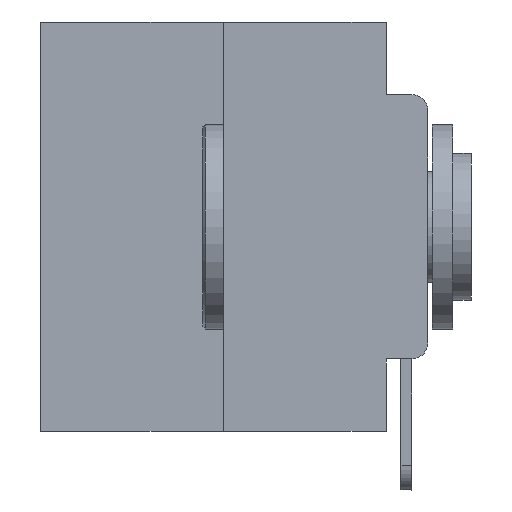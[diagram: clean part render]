
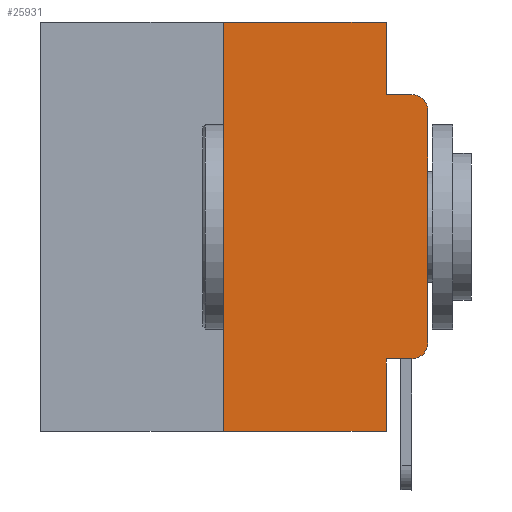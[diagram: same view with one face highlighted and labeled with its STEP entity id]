
A CAD part, left-side view. The second image highlights one B-rep face of the part: STEP entity #25931.
In plain terms, the highlighted planar face has unit normal (-1, 0, 0).
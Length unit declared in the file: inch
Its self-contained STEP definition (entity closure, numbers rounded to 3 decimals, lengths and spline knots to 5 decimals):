
#199 = ORIENTED_EDGE ( 'NONE', *, *, #8933, .F. ) ;
#407 = CARTESIAN_POINT ( 'NONE',  ( 0., 0.051, -0.5 ) ) ;
#454 = CARTESIAN_POINT ( 'NONE',  ( 0., 0.051, 0. ) ) ;
#742 = CARTESIAN_POINT ( 'NONE',  ( 0., 0.051, -0.4115 ) ) ;
#1163 = ORIENTED_EDGE ( 'NONE', *, *, #13655, .T. ) ;
#1267 = DIRECTION ( 'NONE',  ( -1., 0., 0. ) ) ;
#1526 = ORIENTED_EDGE ( 'NONE', *, *, #23392, .T. ) ;
#1685 = VECTOR ( 'NONE', #5749, 39.37008 ) ;
#1769 = DIRECTION ( 'NONE',  ( 0., -1., 0. ) ) ;
#1817 = DIRECTION ( 'NONE',  ( -1., 0., 0. ) ) ;
#2020 = VECTOR ( 'NONE', #12813, 39.37008 ) ;
#2674 = CARTESIAN_POINT ( 'NONE',  ( 0., 0., -0.3915 ) ) ;
#2781 = VERTEX_POINT ( 'NONE', #25508 ) ;
#3095 = EDGE_LOOP ( 'NONE', ( #1526, #18549, #21742, #27456, #24276, #199, #17093, #4495, #1163, #11969 ) ) ;
#3250 = DIRECTION ( 'NONE',  ( 0., 0., -1. ) ) ;
#3511 = CARTESIAN_POINT ( 'NONE',  ( 0., 0., -0.1085 ) ) ;
#3721 = DIRECTION ( 'NONE',  ( 1., 0., 0. ) ) ;
#3898 = VERTEX_POINT ( 'NONE', #15413 ) ;
#4325 = CARTESIAN_POINT ( 'NONE',  ( 0., 0.02, -0.4115 ) ) ;
#4481 = EDGE_CURVE ( 'NONE', #4596, #24447, #20565, .T. ) ;
#4495 = ORIENTED_EDGE ( 'NONE', *, *, #12337, .F. ) ;
#4596 = VERTEX_POINT ( 'NONE', #4325 ) ;
#5749 = DIRECTION ( 'NONE',  ( 0., -1., 0. ) ) ;
#5835 = DIRECTION ( 'NONE',  ( 0., 0., -1. ) ) ;
#5890 = CARTESIAN_POINT ( 'NONE',  ( 0., 0.02, -0.3915 ) ) ;
#6168 = CARTESIAN_POINT ( 'NONE',  ( 0., 0.02, -0.1085 ) ) ;
#6625 = DIRECTION ( 'NONE',  ( 0., 0., 1. ) ) ;
#7272 = VECTOR ( 'NONE', #23406, 39.37008 ) ;
#7619 = CIRCLE ( 'NONE', #13939, 0.02 ) ;
#8236 = LINE ( 'NONE', #26547, #24006 ) ;
#8284 = DIRECTION ( 'NONE',  ( 0., 0., -1. ) ) ;
#8599 = LINE ( 'NONE', #10998, #22497 ) ;
#8933 = EDGE_CURVE ( 'NONE', #17417, #26245, #14877, .T. ) ;
#9037 = LINE ( 'NONE', #454, #23569 ) ;
#9914 = FACE_OUTER_BOUND ( 'NONE', #3095, .T. ) ;
#10382 = DIRECTION ( 'NONE',  ( 0., 0., -1. ) ) ;
#10402 = CARTESIAN_POINT ( 'NONE',  ( 0., 0.051, 0. ) ) ;
#10444 = DIRECTION ( 'NONE',  ( 0., -1., 0. ) ) ;
#10998 = CARTESIAN_POINT ( 'NONE',  ( 0., 0., 0. ) ) ;
#11969 = ORIENTED_EDGE ( 'NONE', *, *, #4481, .T. ) ;
#12337 = EDGE_CURVE ( 'NONE', #20763, #17172, #9037, .T. ) ;
#12813 = DIRECTION ( 'NONE',  ( 0., 0., -1. ) ) ;
#13123 = CARTESIAN_POINT ( 'NONE',  ( 0., 0.473, -0.5 ) ) ;
#13205 = AXIS2_PLACEMENT_3D ( 'NONE', #14280, #3721, #5835 ) ;
#13655 = EDGE_CURVE ( 'NONE', #20763, #4596, #15368, .T. ) ;
#13803 = LINE ( 'NONE', #22341, #1685 ) ;
#13939 = AXIS2_PLACEMENT_3D ( 'NONE', #6168, #1817, #10382 ) ;
#14275 = CARTESIAN_POINT ( 'NONE',  ( 0., 0.051, 0. ) ) ;
#14280 = CARTESIAN_POINT ( 'NONE',  ( 0., 0.473, 0. ) ) ;
#14877 = LINE ( 'NONE', #23133, #7272 ) ;
#15304 = CARTESIAN_POINT ( 'NONE',  ( 0., 0.051, -0.4115 ) ) ;
#15368 = LINE ( 'NONE', #742, #25357 ) ;
#15406 = EDGE_CURVE ( 'NONE', #3898, #2781, #13803, .T. ) ;
#15413 = CARTESIAN_POINT ( 'NONE',  ( 0., 0.051, -0.0885 ) ) ;
#16130 = AXIS2_PLACEMENT_3D ( 'NONE', #5890, #1267, #8284 ) ;
#16665 = PLANE ( 'NONE',  #13205 ) ;
#17017 = LINE ( 'NONE', #10402, #2020 ) ;
#17093 = ORIENTED_EDGE ( 'NONE', *, *, #27704, .T. ) ;
#17172 = VERTEX_POINT ( 'NONE', #407 ) ;
#17417 = VERTEX_POINT ( 'NONE', #22321 ) ;
#17690 = VECTOR ( 'NONE', #10444, 39.37008 ) ;
#17782 = CARTESIAN_POINT ( 'NONE',  ( 0., 0.25, 0. ) ) ;
#18549 = ORIENTED_EDGE ( 'NONE', *, *, #20640, .T. ) ;
#19708 = DIRECTION ( 'NONE',  ( 0., -1., 0. ) ) ;
#20565 = CIRCLE ( 'NONE', #16130, 0.02 ) ;
#20640 = EDGE_CURVE ( 'NONE', #26744, #2781, #7619, .T. ) ;
#20763 = VERTEX_POINT ( 'NONE', #15304 ) ;
#21742 = ORIENTED_EDGE ( 'NONE', *, *, #15406, .F. ) ;
#22321 = CARTESIAN_POINT ( 'NONE',  ( 0., 0.25, -0.5 ) ) ;
#22341 = CARTESIAN_POINT ( 'NONE',  ( 0., 0.051, -0.0885 ) ) ;
#22497 = VECTOR ( 'NONE', #6625, 39.37008 ) ;
#23133 = CARTESIAN_POINT ( 'NONE',  ( 0., 0.25, 0. ) ) ;
#23211 = LINE ( 'NONE', #13123, #17690 ) ;
#23392 = EDGE_CURVE ( 'NONE', #24447, #26744, #8599, .T. ) ;
#23406 = DIRECTION ( 'NONE',  ( 0., 0., 1. ) ) ;
#23569 = VECTOR ( 'NONE', #3250, 39.37008 ) ;
#23985 = VERTEX_POINT ( 'NONE', #14275 ) ;
#24006 = VECTOR ( 'NONE', #1769, 39.37008 ) ;
#24276 = ORIENTED_EDGE ( 'NONE', *, *, #27109, .F. ) ;
#24447 = VERTEX_POINT ( 'NONE', #2674 ) ;
#25357 = VECTOR ( 'NONE', #19708, 39.37008 ) ;
#25508 = CARTESIAN_POINT ( 'NONE',  ( 0., 0.02, -0.0885 ) ) ;
#25931 = ADVANCED_FACE ( 'NONE', ( #9914 ), #16665, .F. ) ;
#26245 = VERTEX_POINT ( 'NONE', #17782 ) ;
#26547 = CARTESIAN_POINT ( 'NONE',  ( 0., 0.473, 0. ) ) ;
#26744 = VERTEX_POINT ( 'NONE', #3511 ) ;
#26955 = EDGE_CURVE ( 'NONE', #23985, #3898, #17017, .T. ) ;
#27109 = EDGE_CURVE ( 'NONE', #26245, #23985, #8236, .T. ) ;
#27456 = ORIENTED_EDGE ( 'NONE', *, *, #26955, .F. ) ;
#27704 = EDGE_CURVE ( 'NONE', #17417, #17172, #23211, .T. ) ;
